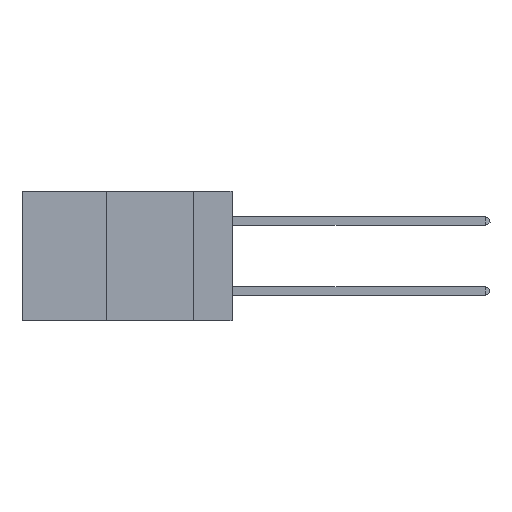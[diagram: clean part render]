
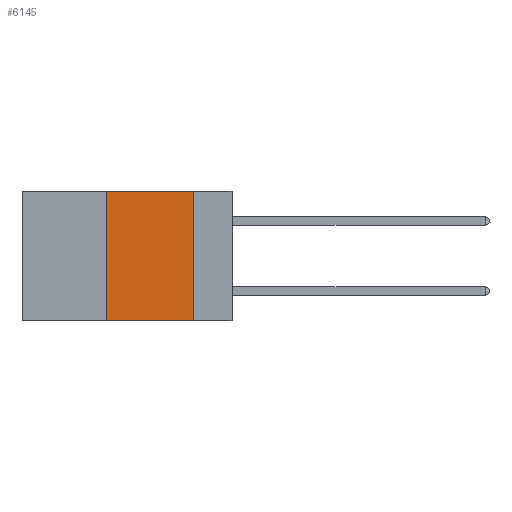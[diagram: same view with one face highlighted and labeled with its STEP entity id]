
A CAD part, left-side view. The second image highlights one B-rep face of the part: STEP entity #6145.
In plain terms, the highlighted planar face has unit normal (-1, 0, 0).
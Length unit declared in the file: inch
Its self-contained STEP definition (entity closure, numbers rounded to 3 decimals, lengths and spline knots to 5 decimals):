
#4 = EDGE_CURVE ( 'NONE', #6717, #1096, #8696, .T. ) ;
#564 = VERTEX_POINT ( 'NONE', #999 ) ;
#957 = DIRECTION ( 'NONE',  ( 0., 0., -1. ) ) ;
#999 = CARTESIAN_POINT ( 'NONE',  ( 0., 0.11, 0. ) ) ;
#1096 = VERTEX_POINT ( 'NONE', #2634 ) ;
#1557 = VECTOR ( 'NONE', #10595, 39.37008 ) ;
#1773 = CARTESIAN_POINT ( 'NONE',  ( 0., 0.11, 0. ) ) ;
#2077 = LINE ( 'NONE', #3105, #1557 ) ;
#2211 = EDGE_CURVE ( 'NONE', #564, #1096, #2877, .T. ) ;
#2287 = CARTESIAN_POINT ( 'NONE',  ( 0., 0.6, 0. ) ) ;
#2386 = EDGE_CURVE ( 'NONE', #9440, #564, #3162, .T. ) ;
#2618 = FACE_OUTER_BOUND ( 'NONE', #2928, .T. ) ;
#2634 = CARTESIAN_POINT ( 'NONE',  ( 0., 0.11, -0.37 ) ) ;
#2877 = LINE ( 'NONE', #1773, #10691 ) ;
#2928 = EDGE_LOOP ( 'NONE', ( #6123, #8932, #6383, #6427 ) ) ;
#3105 = CARTESIAN_POINT ( 'NONE',  ( 0., 0.36, 0. ) ) ;
#3162 = LINE ( 'NONE', #5595, #9553 ) ;
#3178 = AXIS2_PLACEMENT_3D ( 'NONE', #2287, #10538, #6436 ) ;
#5137 = VECTOR ( 'NONE', #8717, 39.37008 ) ;
#5520 = CARTESIAN_POINT ( 'NONE',  ( 0., 0.6, -0.37 ) ) ;
#5595 = CARTESIAN_POINT ( 'NONE',  ( 0., 0.6, 0. ) ) ;
#5637 = CARTESIAN_POINT ( 'NONE',  ( 0., 0.36, -0.37 ) ) ;
#5652 = CARTESIAN_POINT ( 'NONE',  ( 0., 0.36, 0. ) ) ;
#6123 = ORIENTED_EDGE ( 'NONE', *, *, #2211, .F. ) ;
#6145 = ADVANCED_FACE ( 'NONE', ( #2618 ), #8091, .F. ) ;
#6383 = ORIENTED_EDGE ( 'NONE', *, *, #6819, .F. ) ;
#6427 = ORIENTED_EDGE ( 'NONE', *, *, #4, .T. ) ;
#6436 = DIRECTION ( 'NONE',  ( 0., 0., -1. ) ) ;
#6717 = VERTEX_POINT ( 'NONE', #5637 ) ;
#6819 = EDGE_CURVE ( 'NONE', #6717, #9440, #2077, .T. ) ;
#8091 = PLANE ( 'NONE',  #3178 ) ;
#8696 = LINE ( 'NONE', #5520, #5137 ) ;
#8717 = DIRECTION ( 'NONE',  ( 0., -1., 0. ) ) ;
#8932 = ORIENTED_EDGE ( 'NONE', *, *, #2386, .F. ) ;
#9440 = VERTEX_POINT ( 'NONE', #5652 ) ;
#9553 = VECTOR ( 'NONE', #9764, 39.37008 ) ;
#9764 = DIRECTION ( 'NONE',  ( 0., -1., 0. ) ) ;
#10538 = DIRECTION ( 'NONE',  ( 1., 0., 0. ) ) ;
#10595 = DIRECTION ( 'NONE',  ( 0., 0., 1. ) ) ;
#10691 = VECTOR ( 'NONE', #957, 39.37008 ) ;
